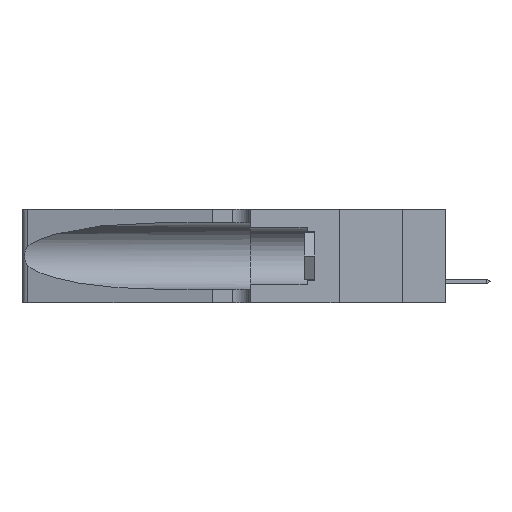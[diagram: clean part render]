
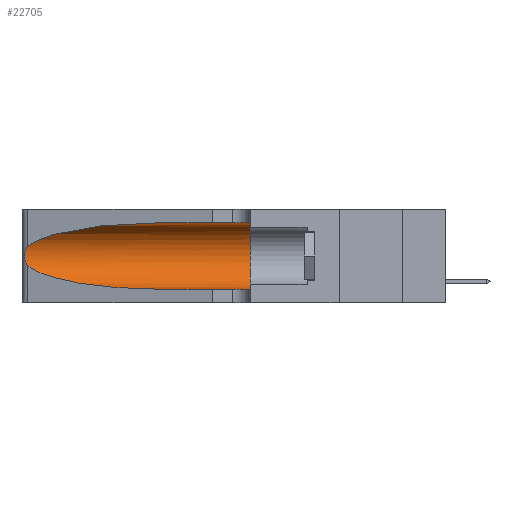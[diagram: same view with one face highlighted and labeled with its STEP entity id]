
A CAD part, left-side view. The second image highlights one B-rep face of the part: STEP entity #22705.
In plain terms, the highlighted cylindrical face has radius 3.308 mm (diameter 6.617 mm), a partial arc.
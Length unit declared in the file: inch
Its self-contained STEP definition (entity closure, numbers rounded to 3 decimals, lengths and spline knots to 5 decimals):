
#727 = VERTEX_POINT ( 'NONE', #26274 ) ;
#1112 = CARTESIAN_POINT ( 'NONE',  ( 0.25487, 1.22718, 0.22369 ) ) ;
#1255 = CARTESIAN_POINT ( 'NONE',  ( 0.25555, 1.22993, 0.14849 ) ) ;
#2352 = CARTESIAN_POINT ( 'NONE',  ( 0.25639, 1.23184, 0.21858 ) ) ;
#2632 = CARTESIAN_POINT ( 'NONE',  ( 0.25854, 1.2359, 0.20912 ) ) ;
#2730 = ORIENTED_EDGE ( 'NONE', *, *, #6858, .F. ) ;
#3254 = CARTESIAN_POINT ( 'NONE',  ( 0.2373, 1.15595, 0.28018 ) ) ;
#3468 = CARTESIAN_POINT ( 'NONE',  ( 0.1305, 1.61858, 0.05475 ) ) ;
#3474 = VERTEX_POINT ( 'NONE', #24493 ) ;
#3665 = VERTEX_POINT ( 'NONE', #12975 ) ;
#4958 = CARTESIAN_POINT ( 'NONE',  ( 0.25487, 1.22718, 0.22369 ) ) ;
#5234 = CARTESIAN_POINT ( 'NONE',  ( 0.1305, 0.35, 0.31525 ) ) ;
#5582 = CARTESIAN_POINT ( 'NONE',  ( 0.2373, 1.15595, 0.08982 ) ) ;
#5893 = CARTESIAN_POINT ( 'NONE',  ( 0.25789, 1.23486, 0.15765 ) ) ;
#6777 = CARTESIAN_POINT ( 'NONE',  ( 0.26017, 1.23833, 0.17102 ) ) ;
#6858 = EDGE_CURVE ( 'NONE', #15068, #13577, #11219, .T. ) ;
#7221 = DIRECTION ( 'NONE',  ( 0., 0., -1. ) ) ;
#7686 = CARTESIAN_POINT ( 'NONE',  ( 0.1305, 0.72297, 0.31525 ) ) ;
#7701 = CARTESIAN_POINT ( 'NONE',  ( 0.25487, 1.22718, 0.14631 ) ) ;
#7942 = DIRECTION ( 'NONE',  ( 0., 1., 0. ) ) ;
#8401 = LINE ( 'NONE', #3468, #9426 ) ;
#8551 = CARTESIAN_POINT ( 'NONE',  ( 0.25487, 1.22718, 0.22369 ) ) ;
#8837 = VECTOR ( 'NONE', #17867, 39.37008 ) ;
#9305 = CIRCLE ( 'NONE', #25725, 0.13025 ) ;
#9426 = VECTOR ( 'NONE', #18970, 39.37008 ) ;
#9770 = EDGE_CURVE ( 'NONE', #3665, #3474, #8401, .T. ) ;
#10324 = CARTESIAN_POINT ( 'NONE',  ( 0.25856, 1.23593, 0.16098 ) ) ;
#10333 = VERTEX_POINT ( 'NONE', #8551 ) ;
#10491 = ORIENTED_EDGE ( 'NONE', *, *, #27832, .F. ) ;
#11219 = LINE ( 'NONE', #22194, #8837 ) ;
#11224 = ORIENTED_EDGE ( 'NONE', *, *, #9770, .T. ) ;
#11733 = EDGE_CURVE ( 'NONE', #15068, #10333, #19141, .T. ) ;
#12143 = CARTESIAN_POINT ( 'NONE',  ( 0.25639, 1.23186, 0.15144 ) ) ;
#12180 = ORIENTED_EDGE ( 'NONE', *, *, #15184, .T. ) ;
#12975 = CARTESIAN_POINT ( 'NONE',  ( 0.1305, 0.72297, 0.05475 ) ) ;
#13577 = VERTEX_POINT ( 'NONE', #5234 ) ;
#13604 = CARTESIAN_POINT ( 'NONE',  ( 0.25787, 1.23484, 0.2124 ) ) ;
#14194 = CARTESIAN_POINT ( 'NONE',  ( 0.18966, 0.96281, 0.31525 ) ) ;
#14309 = CARTESIAN_POINT ( 'NONE',  ( 0.1305, 0.72297, 0.05475 ) ) ;
#15068 = VERTEX_POINT ( 'NONE', #27918 ) ;
#15078 = AXIS2_PLACEMENT_3D ( 'NONE', #20444, #25156, #7221 ) ;
#15184 = EDGE_CURVE ( 'NONE', #10333, #727, #23558, .T. ) ;
#17563 =( BOUNDED_CURVE ( )  B_SPLINE_CURVE ( 3, ( #7701, #5582, #18601, #14309 ),
 .UNSPECIFIED., .F., .F. ) 
 B_SPLINE_CURVE_WITH_KNOTS ( ( 4, 4 ),
 ( 3.44316, 4.71239 ),
 .UNSPECIFIED. ) 
 CURVE ( )  GEOMETRIC_REPRESENTATION_ITEM ( )  RATIONAL_B_SPLINE_CURVE ( ( 1., 0.87, 0.87, 1. ) ) 
 REPRESENTATION_ITEM ( '' )  );
#17867 = DIRECTION ( 'NONE',  ( 0., -1., 0. ) ) ;
#18601 = CARTESIAN_POINT ( 'NONE',  ( 0.18966, 0.96281, 0.05475 ) ) ;
#18647 = DIRECTION ( 'NONE',  ( 0., 0., 1. ) ) ;
#18970 = DIRECTION ( 'NONE',  ( 0., -1., 0. ) ) ;
#19141 =( BOUNDED_CURVE ( )  B_SPLINE_CURVE ( 3, ( #7686, #14194, #3254, #1112 ),
 .UNSPECIFIED., .F., .F. ) 
 B_SPLINE_CURVE_WITH_KNOTS ( ( 4, 4 ),
 ( 1.5708, 2.84003 ),
 .UNSPECIFIED. ) 
 CURVE ( )  GEOMETRIC_REPRESENTATION_ITEM ( )  RATIONAL_B_SPLINE_CURVE ( ( 1., 0.87, 0.87, 1. ) ) 
 REPRESENTATION_ITEM ( '' )  );
#19912 = CARTESIAN_POINT ( 'NONE',  ( 0.25555, 1.22994, 0.2215 ) ) ;
#20444 = CARTESIAN_POINT ( 'NONE',  ( 0.1305, 1.61858, 0.185 ) ) ;
#20946 = CARTESIAN_POINT ( 'NONE',  ( 0.25487, 1.22718, 0.14631 ) ) ;
#20951 = CARTESIAN_POINT ( 'NONE',  ( 0.1305, 0.35, 0.185 ) ) ;
#22194 = CARTESIAN_POINT ( 'NONE',  ( 0.1305, 1.61858, 0.31525 ) ) ;
#22209 = CARTESIAN_POINT ( 'NONE',  ( 0.26018, 1.23835, 0.19895 ) ) ;
#22705 = ADVANCED_FACE ( 'NONE', ( #23685 ), #25072, .F. ) ;
#23558 = B_SPLINE_CURVE_WITH_KNOTS ( 'NONE', 3,
 ( #4958, #19912, #2352, #13604, #2632, #22209, #24725, #24623, #6777, #10324, #5893, #12143, #1255, #20946 ),
 .UNSPECIFIED., .F., .F.,
 ( 4, 2, 2, 2, 2, 2, 4 ),
 ( 0., 0.00027, 0.00053, 0.00107, 0.0016, 0.00187, 0.00214 ),
 .UNSPECIFIED. ) ;
#23685 = FACE_OUTER_BOUND ( 'NONE', #23804, .T. ) ;
#23804 = EDGE_LOOP ( 'NONE', ( #26259, #12180, #28063, #11224, #10491, #2730 ) ) ;
#24493 = CARTESIAN_POINT ( 'NONE',  ( 0.1305, 0.35, 0.05475 ) ) ;
#24623 = CARTESIAN_POINT ( 'NONE',  ( 0.26075, 1.23896, 0.178 ) ) ;
#24725 = CARTESIAN_POINT ( 'NONE',  ( 0.26075, 1.23896, 0.19203 ) ) ;
#24963 = EDGE_CURVE ( 'NONE', #727, #3665, #17563, .T. ) ;
#25072 = CYLINDRICAL_SURFACE ( 'NONE', #15078, 0.13025 ) ;
#25156 = DIRECTION ( 'NONE',  ( 0., -1., 0. ) ) ;
#25725 = AXIS2_PLACEMENT_3D ( 'NONE', #20951, #7942, #18647 ) ;
#26259 = ORIENTED_EDGE ( 'NONE', *, *, #11733, .T. ) ;
#26274 = CARTESIAN_POINT ( 'NONE',  ( 0.25487, 1.22718, 0.14631 ) ) ;
#27832 = EDGE_CURVE ( 'NONE', #13577, #3474, #9305, .T. ) ;
#27918 = CARTESIAN_POINT ( 'NONE',  ( 0.1305, 0.72297, 0.31525 ) ) ;
#28063 = ORIENTED_EDGE ( 'NONE', *, *, #24963, .T. ) ;
